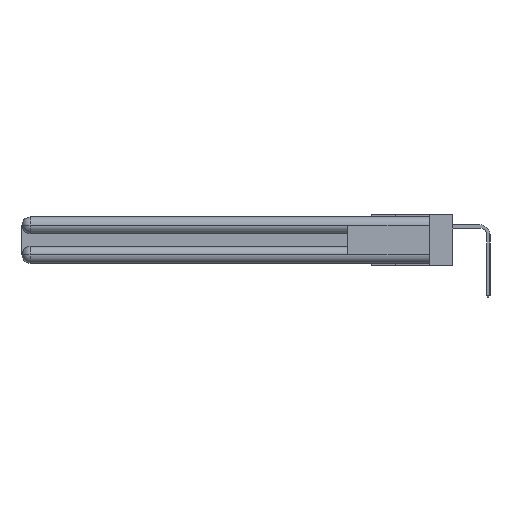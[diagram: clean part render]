
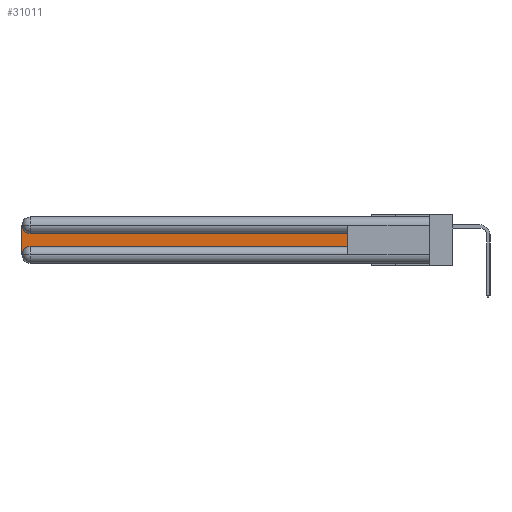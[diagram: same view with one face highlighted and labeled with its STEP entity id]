
A CAD part, left-side view. The second image highlights one B-rep face of the part: STEP entity #31011.
In plain terms, the highlighted planar face has unit normal (-1, 0, 0).
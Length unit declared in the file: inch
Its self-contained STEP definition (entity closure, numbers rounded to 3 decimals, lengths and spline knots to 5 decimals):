
#134 = CARTESIAN_POINT ( 'NONE',  ( 0.075, 2.94, -0.0625 ) ) ;
#167 = CIRCLE ( 'NONE', #6892, 0.06 ) ;
#1200 = CARTESIAN_POINT ( 'NONE',  ( 0.075, 0.6, -0.2175 ) ) ;
#1284 = CARTESIAN_POINT ( 'NONE',  ( 0.075, 3., -0.0625 ) ) ;
#2077 = CIRCLE ( 'NONE', #13959, 0.06 ) ;
#2480 = DIRECTION ( 'NONE',  ( 0., 0., -1. ) ) ;
#3805 = EDGE_CURVE ( 'NONE', #9669, #7415, #5254, .T. ) ;
#3954 = ORIENTED_EDGE ( 'NONE', *, *, #22309, .T. ) ;
#4759 = VECTOR ( 'NONE', #29327, 39.37008 ) ;
#5039 = DIRECTION ( 'NONE',  ( 0., 0., -1. ) ) ;
#5254 = LINE ( 'NONE', #9972, #21593 ) ;
#6892 = AXIS2_PLACEMENT_3D ( 'NONE', #7276, #18501, #28720 ) ;
#7276 = CARTESIAN_POINT ( 'NONE',  ( 0.075, 2.94, -0.2775 ) ) ;
#7287 = DIRECTION ( 'NONE',  ( 1., 0., 0. ) ) ;
#7415 = VERTEX_POINT ( 'NONE', #7845 ) ;
#7845 = CARTESIAN_POINT ( 'NONE',  ( 0.075, 0.6, -0.2175 ) ) ;
#7995 = CARTESIAN_POINT ( 'NONE',  ( 0.075, 3., -0.2175 ) ) ;
#8986 = DIRECTION ( 'NONE',  ( 1., 0., 0. ) ) ;
#9512 = VECTOR ( 'NONE', #2480, 39.37008 ) ;
#9643 = EDGE_CURVE ( 'NONE', #7415, #13609, #25898, .T. ) ;
#9669 = VERTEX_POINT ( 'NONE', #33426 ) ;
#9802 = EDGE_CURVE ( 'NONE', #19239, #30369, #10338, .T. ) ;
#9972 = CARTESIAN_POINT ( 'NONE',  ( 0.075, 0.6, -0.2175 ) ) ;
#10338 = LINE ( 'NONE', #7995, #9512 ) ;
#11850 = LINE ( 'NONE', #21248, #4759 ) ;
#12942 = EDGE_CURVE ( 'NONE', #30369, #9669, #167, .T. ) ;
#13096 = ORIENTED_EDGE ( 'NONE', *, *, #9643, .T. ) ;
#13609 = VERTEX_POINT ( 'NONE', #29676 ) ;
#13959 = AXIS2_PLACEMENT_3D ( 'NONE', #134, #8986, #5039 ) ;
#14731 = VERTEX_POINT ( 'NONE', #33921 ) ;
#15257 = DIRECTION ( 'NONE',  ( 0., 0., -1. ) ) ;
#15958 = FACE_OUTER_BOUND ( 'NONE', #18194, .T. ) ;
#18194 = EDGE_LOOP ( 'NONE', ( #3954, #33453, #29901, #22413, #19269, #13096 ) ) ;
#18501 = DIRECTION ( 'NONE',  ( 1., 0., 0. ) ) ;
#19239 = VERTEX_POINT ( 'NONE', #1284 ) ;
#19269 = ORIENTED_EDGE ( 'NONE', *, *, #3805, .T. ) ;
#19772 = EDGE_CURVE ( 'NONE', #14731, #19239, #2077, .T. ) ;
#20440 = DIRECTION ( 'NONE',  ( 0., -1., 0. ) ) ;
#20653 = CARTESIAN_POINT ( 'NONE',  ( 0.075, 3., -0.1225 ) ) ;
#21248 = CARTESIAN_POINT ( 'NONE',  ( 0.075, 0.6, -0.1225 ) ) ;
#21593 = VECTOR ( 'NONE', #20440, 39.37008 ) ;
#22309 = EDGE_CURVE ( 'NONE', #13609, #14731, #11850, .T. ) ;
#22413 = ORIENTED_EDGE ( 'NONE', *, *, #12942, .T. ) ;
#25898 = LINE ( 'NONE', #1200, #28003 ) ;
#28003 = VECTOR ( 'NONE', #30833, 39.37008 ) ;
#28720 = DIRECTION ( 'NONE',  ( 0., 0., -1. ) ) ;
#29327 = DIRECTION ( 'NONE',  ( 0., 1., 0. ) ) ;
#29676 = CARTESIAN_POINT ( 'NONE',  ( 0.075, 0.6, -0.1225 ) ) ;
#29901 = ORIENTED_EDGE ( 'NONE', *, *, #9802, .T. ) ;
#29948 = AXIS2_PLACEMENT_3D ( 'NONE', #20653, #7287, #15257 ) ;
#29972 = CARTESIAN_POINT ( 'NONE',  ( 0.075, 3., -0.2775 ) ) ;
#30369 = VERTEX_POINT ( 'NONE', #29972 ) ;
#30833 = DIRECTION ( 'NONE',  ( 0., 0., 1. ) ) ;
#31011 = ADVANCED_FACE ( 'NONE', ( #15958 ), #31696, .F. ) ;
#31696 = PLANE ( 'NONE',  #29948 ) ;
#33426 = CARTESIAN_POINT ( 'NONE',  ( 0.075, 2.94, -0.2175 ) ) ;
#33453 = ORIENTED_EDGE ( 'NONE', *, *, #19772, .T. ) ;
#33921 = CARTESIAN_POINT ( 'NONE',  ( 0.075, 2.94, -0.1225 ) ) ;
